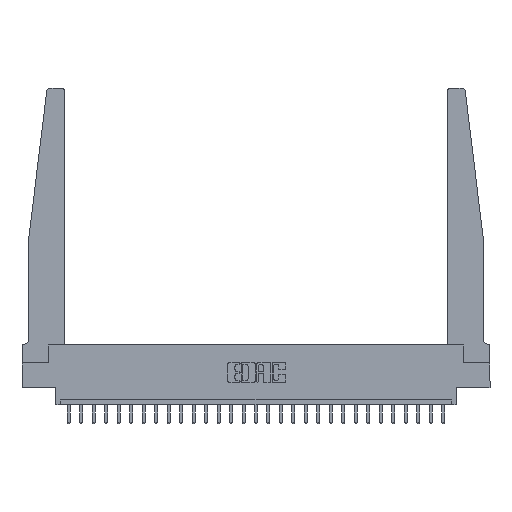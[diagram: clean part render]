
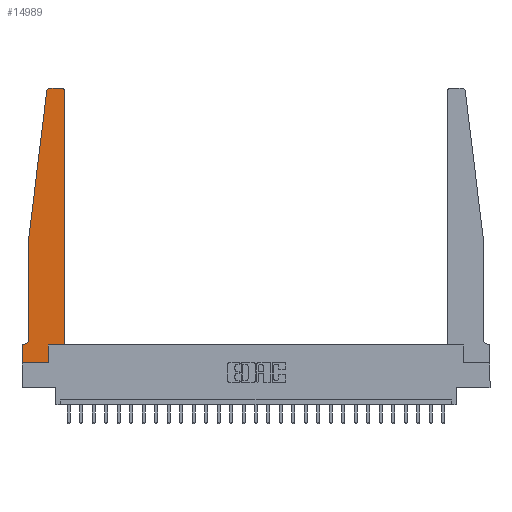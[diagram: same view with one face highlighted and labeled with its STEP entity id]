
A CAD part, top view. The second image highlights one B-rep face of the part: STEP entity #14989.
In plain terms, the highlighted planar face has unit normal (0, 0, 1).
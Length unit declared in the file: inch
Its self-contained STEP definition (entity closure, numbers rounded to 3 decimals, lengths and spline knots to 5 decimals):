
#1366 = ORIENTED_EDGE ( 'NONE', *, *, #21814, .T. ) ;
#1406 = CARTESIAN_POINT ( 'NONE',  ( 0.065, 1.25, 0.37 ) ) ;
#1463 = DIRECTION ( 'NONE',  ( -0.122, -0.992, 0. ) ) ;
#2126 = CARTESIAN_POINT ( 'NONE',  ( 0.395, 2.72, 0.37 ) ) ;
#2213 = DIRECTION ( 'NONE',  ( 0., 0., 1. ) ) ;
#2372 = AXIS2_PLACEMENT_3D ( 'NONE', #16106, #2396, #14164 ) ;
#2396 = DIRECTION ( 'NONE',  ( 0., 0., -1. ) ) ;
#2406 = FACE_OUTER_BOUND ( 'NONE', #4524, .T. ) ;
#2525 = VECTOR ( 'NONE', #6340, 39.37008 ) ;
#2779 = EDGE_CURVE ( 'NONE', #14529, #20816, #25528, .T. ) ;
#2885 = EDGE_CURVE ( 'NONE', #5431, #5116, #7767, .T. ) ;
#2943 = DIRECTION ( 'NONE',  ( 0., 1., 0. ) ) ;
#2964 = EDGE_CURVE ( 'NONE', #24389, #14529, #4369, .T. ) ;
#3352 = CARTESIAN_POINT ( 'NONE',  ( 0.065, 0.2375, 0.37 ) ) ;
#3821 = EDGE_CURVE ( 'NONE', #8025, #15222, #5876, .T. ) ;
#4071 = ORIENTED_EDGE ( 'NONE', *, *, #2964, .T. ) ;
#4293 = VECTOR ( 'NONE', #5511, 39.37008 ) ;
#4311 = DIRECTION ( 'NONE',  ( 1., 0., 0. ) ) ;
#4369 = LINE ( 'NONE', #1406, #14253 ) ;
#4524 = EDGE_LOOP ( 'NONE', ( #9943, #10535, #11908, #4071, #16035, #7955, #4593, #14213, #1366, #11752, #16383, #9427 ) ) ;
#4593 = ORIENTED_EDGE ( 'NONE', *, *, #11391, .T. ) ;
#4810 = VERTEX_POINT ( 'NONE', #20788 ) ;
#4888 = CARTESIAN_POINT ( 'NONE',  ( 0.27653, 2.75, 0.37 ) ) ;
#4924 = CARTESIAN_POINT ( 'NONE',  ( 0.015, 0.1875, 0.37 ) ) ;
#4931 = VECTOR ( 'NONE', #2943, 39.37008 ) ;
#5116 = VERTEX_POINT ( 'NONE', #13336 ) ;
#5126 = EDGE_CURVE ( 'NONE', #24362, #7164, #15727, .T. ) ;
#5431 = VERTEX_POINT ( 'NONE', #16847 ) ;
#5511 = DIRECTION ( 'NONE',  ( -1., 0., 0. ) ) ;
#5876 = CIRCLE ( 'NONE', #18346, 0.03 ) ;
#5933 = CARTESIAN_POINT ( 'NONE',  ( 0., 0., 0.37 ) ) ;
#6245 = EDGE_CURVE ( 'NONE', #23909, #4810, #11527, .T. ) ;
#6340 = DIRECTION ( 'NONE',  ( 1., 0., 0. ) ) ;
#6661 = LINE ( 'NONE', #16428, #24053 ) ;
#7000 = CARTESIAN_POINT ( 'NONE',  ( 0., 0.1875, 0.37 ) ) ;
#7056 = LINE ( 'NONE', #13364, #4293 ) ;
#7164 = VERTEX_POINT ( 'NONE', #8803 ) ;
#7168 = LINE ( 'NONE', #25073, #20558 ) ;
#7767 = LINE ( 'NONE', #5933, #2525 ) ;
#7779 = VERTEX_POINT ( 'NONE', #12509 ) ;
#7955 = ORIENTED_EDGE ( 'NONE', *, *, #9526, .T. ) ;
#8025 = VERTEX_POINT ( 'NONE', #4888 ) ;
#8201 = DIRECTION ( 'NONE',  ( 0., 1., 0. ) ) ;
#8803 = CARTESIAN_POINT ( 'NONE',  ( 0.425, 0.18, 0.37 ) ) ;
#9276 = CARTESIAN_POINT ( 'NONE',  ( 0.2605, 0.18, 0.37 ) ) ;
#9382 = LINE ( 'NONE', #12829, #14029 ) ;
#9427 = ORIENTED_EDGE ( 'NONE', *, *, #6245, .T. ) ;
#9526 = EDGE_CURVE ( 'NONE', #20816, #7779, #7056, .T. ) ;
#9943 = ORIENTED_EDGE ( 'NONE', *, *, #18276, .T. ) ;
#10535 = ORIENTED_EDGE ( 'NONE', *, *, #3821, .T. ) ;
#11391 = EDGE_CURVE ( 'NONE', #7779, #5431, #6661, .T. ) ;
#11527 = CIRCLE ( 'NONE', #16560, 0.03 ) ;
#11666 = DIRECTION ( 'NONE',  ( 0., -1., 0. ) ) ;
#11752 = ORIENTED_EDGE ( 'NONE', *, *, #5126, .T. ) ;
#11908 = ORIENTED_EDGE ( 'NONE', *, *, #19088, .T. ) ;
#11911 = CARTESIAN_POINT ( 'NONE',  ( 0.425, 2.72, 0.37 ) ) ;
#12509 = CARTESIAN_POINT ( 'NONE',  ( 0., 0.1875, 0.37 ) ) ;
#12748 = DIRECTION ( 'NONE',  ( -1., 0., 0. ) ) ;
#12829 = CARTESIAN_POINT ( 'NONE',  ( 0.25, 2.75, 0.37 ) ) ;
#12896 = DIRECTION ( 'NONE',  ( 1., 0., 0. ) ) ;
#13336 = CARTESIAN_POINT ( 'NONE',  ( 0.2605, 0., 0.37 ) ) ;
#13364 = CARTESIAN_POINT ( 'NONE',  ( 0.065, 0.1875, 0.37 ) ) ;
#14029 = VECTOR ( 'NONE', #12748, 39.37008 ) ;
#14069 = DIRECTION ( 'NONE',  ( 1., 0., 0. ) ) ;
#14164 = DIRECTION ( 'NONE',  ( -1., 0., 0. ) ) ;
#14213 = ORIENTED_EDGE ( 'NONE', *, *, #2885, .T. ) ;
#14253 = VECTOR ( 'NONE', #11666, 39.37008 ) ;
#14529 = VERTEX_POINT ( 'NONE', #3352 ) ;
#14989 = ADVANCED_FACE ( 'NONE', ( #2406 ), #24729, .T. ) ;
#15110 = VECTOR ( 'NONE', #8201, 39.37008 ) ;
#15222 = VERTEX_POINT ( 'NONE', #16961 ) ;
#15727 = LINE ( 'NONE', #21526, #23795 ) ;
#16009 = DIRECTION ( 'NONE',  ( 0., 0., 1. ) ) ;
#16035 = ORIENTED_EDGE ( 'NONE', *, *, #2779, .T. ) ;
#16106 = CARTESIAN_POINT ( 'NONE',  ( 0.015, 0.2375, 0.37 ) ) ;
#16246 = DIRECTION ( 'NONE',  ( 0., -1., 0. ) ) ;
#16383 = ORIENTED_EDGE ( 'NONE', *, *, #21887, .T. ) ;
#16428 = CARTESIAN_POINT ( 'NONE',  ( 0., 0., 0.37 ) ) ;
#16560 = AXIS2_PLACEMENT_3D ( 'NONE', #2126, #16009, #14069 ) ;
#16847 = CARTESIAN_POINT ( 'NONE',  ( 0., 0., 0.37 ) ) ;
#16961 = CARTESIAN_POINT ( 'NONE',  ( 0.24675, 2.72367, 0.37 ) ) ;
#17646 = DIRECTION ( 'NONE',  ( 1., 0., 0. ) ) ;
#17933 = CARTESIAN_POINT ( 'NONE',  ( 0.27653, 2.72, 0.37 ) ) ;
#18276 = EDGE_CURVE ( 'NONE', #4810, #8025, #9382, .T. ) ;
#18346 = AXIS2_PLACEMENT_3D ( 'NONE', #17933, #2213, #4311 ) ;
#18837 = DIRECTION ( 'NONE',  ( 0., 0., 1. ) ) ;
#19088 = EDGE_CURVE ( 'NONE', #15222, #24389, #7168, .T. ) ;
#19196 = LINE ( 'NONE', #22172, #15110 ) ;
#20558 = VECTOR ( 'NONE', #1463, 39.37008 ) ;
#20788 = CARTESIAN_POINT ( 'NONE',  ( 0.395, 2.75, 0.37 ) ) ;
#20816 = VERTEX_POINT ( 'NONE', #4924 ) ;
#21441 = CARTESIAN_POINT ( 'NONE',  ( 0.065, 1.25, 0.37 ) ) ;
#21526 = CARTESIAN_POINT ( 'NONE',  ( 0.425, 0.18, 0.37 ) ) ;
#21814 = EDGE_CURVE ( 'NONE', #5116, #24362, #19196, .T. ) ;
#21887 = EDGE_CURVE ( 'NONE', #7164, #23909, #24451, .T. ) ;
#22172 = CARTESIAN_POINT ( 'NONE',  ( 0.2605, 0.18, 0.37 ) ) ;
#22453 = CARTESIAN_POINT ( 'NONE',  ( 0.425, 0.18, 0.37 ) ) ;
#23795 = VECTOR ( 'NONE', #17646, 39.37008 ) ;
#23909 = VERTEX_POINT ( 'NONE', #11911 ) ;
#24044 = AXIS2_PLACEMENT_3D ( 'NONE', #7000, #18837, #12896 ) ;
#24053 = VECTOR ( 'NONE', #16246, 39.37008 ) ;
#24362 = VERTEX_POINT ( 'NONE', #9276 ) ;
#24389 = VERTEX_POINT ( 'NONE', #21441 ) ;
#24451 = LINE ( 'NONE', #22453, #4931 ) ;
#24729 = PLANE ( 'NONE',  #24044 ) ;
#25073 = CARTESIAN_POINT ( 'NONE',  ( 0.065, 1.25, 0.37 ) ) ;
#25528 = CIRCLE ( 'NONE', #2372, 0.05 ) ;
